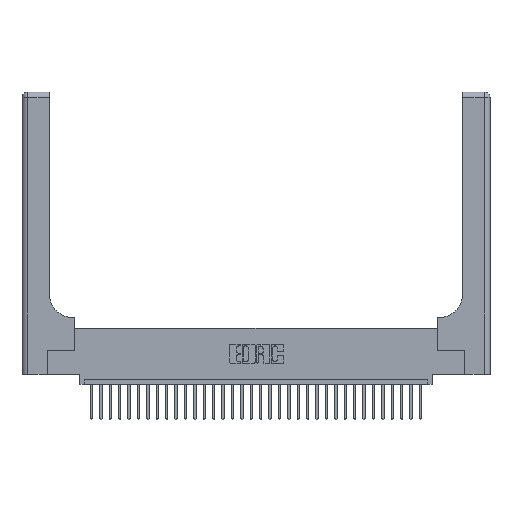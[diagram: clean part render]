
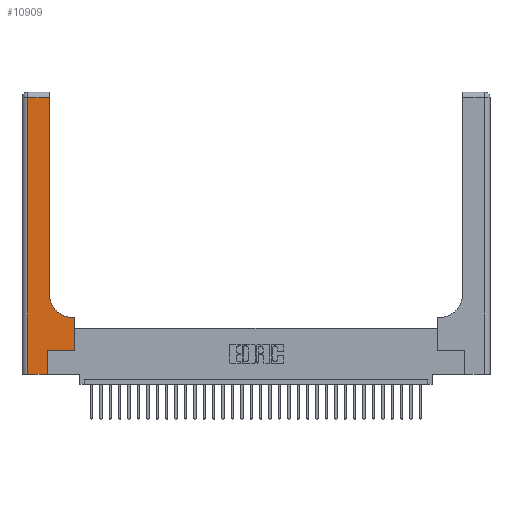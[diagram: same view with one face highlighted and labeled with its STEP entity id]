
A CAD part, top view. The second image highlights one B-rep face of the part: STEP entity #10909.
In plain terms, the highlighted planar face has unit normal (0, 0, 1).
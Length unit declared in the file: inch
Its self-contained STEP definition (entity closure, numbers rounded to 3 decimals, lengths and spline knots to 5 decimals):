
#302 = DIRECTION ( 'NONE',  ( -1., 0., 0. ) ) ;
#313 = CARTESIAN_POINT ( 'NONE',  ( 0., 0., 0.37 ) ) ;
#1082 = DIRECTION ( 'NONE',  ( 0., 1., 0. ) ) ;
#1870 = DIRECTION ( 'NONE',  ( 0., 0., -1. ) ) ;
#2086 = PLANE ( 'NONE',  #30559 ) ;
#2794 = DIRECTION ( 'NONE',  ( 1., 0., 0. ) ) ;
#3475 = VECTOR ( 'NONE', #12350, 39.37008 ) ;
#3550 = VERTEX_POINT ( 'NONE', #29583 ) ;
#3606 = EDGE_CURVE ( 'NONE', #26972, #3550, #19861, .T. ) ;
#3773 = EDGE_CURVE ( 'NONE', #23909, #29468, #15411, .T. ) ;
#4228 = ORIENTED_EDGE ( 'NONE', *, *, #3606, .T. ) ;
#4654 = CARTESIAN_POINT ( 'NONE',  ( 0., 3., 0.37 ) ) ;
#5030 = ORIENTED_EDGE ( 'NONE', *, *, #11536, .T. ) ;
#5395 = DIRECTION ( 'NONE',  ( 0., 1., 0. ) ) ;
#5443 = VECTOR ( 'NONE', #5395, 39.37008 ) ;
#6103 = ORIENTED_EDGE ( 'NONE', *, *, #27163, .T. ) ;
#7341 = DIRECTION ( 'NONE',  ( -1., 0., 0. ) ) ;
#7706 = CARTESIAN_POINT ( 'NONE',  ( 0.269, 0.25, 0.37 ) ) ;
#8297 = CARTESIAN_POINT ( 'NONE',  ( 0.2915, 0.85, 0.37 ) ) ;
#8334 = CARTESIAN_POINT ( 'NONE',  ( 0.5415, 0.85, 0.37 ) ) ;
#8568 = CARTESIAN_POINT ( 'NONE',  ( 0.269, 0., 0.37 ) ) ;
#9108 = CARTESIAN_POINT ( 'NONE',  ( 0.06, 2.94, 0.37 ) ) ;
#9477 = VECTOR ( 'NONE', #7341, 39.37008 ) ;
#9943 = LINE ( 'NONE', #11959, #5443 ) ;
#10534 = LINE ( 'NONE', #15689, #28540 ) ;
#10909 = ADVANCED_FACE ( 'NONE', ( #15616 ), #2086, .F. ) ;
#11064 = VECTOR ( 'NONE', #1082, 39.37008 ) ;
#11536 = EDGE_CURVE ( 'NONE', #12377, #16761, #32868, .T. ) ;
#11605 = EDGE_CURVE ( 'NONE', #32882, #12377, #17578, .T. ) ;
#11951 = LINE ( 'NONE', #15032, #3475 ) ;
#11959 = CARTESIAN_POINT ( 'NONE',  ( 0.269, 0., 0.37 ) ) ;
#12200 = EDGE_CURVE ( 'NONE', #17637, #17462, #11951, .T. ) ;
#12301 = CARTESIAN_POINT ( 'NONE',  ( 0.5585, 0.25, 0.37 ) ) ;
#12350 = DIRECTION ( 'NONE',  ( 1., 0., 0. ) ) ;
#12377 = VERTEX_POINT ( 'NONE', #21167 ) ;
#12618 = EDGE_CURVE ( 'NONE', #16761, #17637, #9943, .T. ) ;
#14243 = EDGE_CURVE ( 'NONE', #3550, #23909, #27149, .T. ) ;
#15032 = CARTESIAN_POINT ( 'NONE',  ( 0.269, 0.25, 0.37 ) ) ;
#15411 = LINE ( 'NONE', #21137, #20235 ) ;
#15616 = FACE_OUTER_BOUND ( 'NONE', #30904, .T. ) ;
#15689 = CARTESIAN_POINT ( 'NONE',  ( 0., 2.94, 0.37 ) ) ;
#15987 = CARTESIAN_POINT ( 'NONE',  ( 0.5585, 0.25, 0.37 ) ) ;
#16761 = VERTEX_POINT ( 'NONE', #8568 ) ;
#17462 = VERTEX_POINT ( 'NONE', #12301 ) ;
#17578 = LINE ( 'NONE', #23060, #28810 ) ;
#17637 = VERTEX_POINT ( 'NONE', #7706 ) ;
#17862 = LINE ( 'NONE', #15987, #11064 ) ;
#19861 = LINE ( 'NONE', #27658, #9477 ) ;
#20159 = ORIENTED_EDGE ( 'NONE', *, *, #29203, .T. ) ;
#20235 = VECTOR ( 'NONE', #30074, 39.37008 ) ;
#20959 = DIRECTION ( 'NONE',  ( 0., 0., -1. ) ) ;
#21137 = CARTESIAN_POINT ( 'NONE',  ( 0.2915, 3., 0.37 ) ) ;
#21167 = CARTESIAN_POINT ( 'NONE',  ( 0.06, 0., 0.37 ) ) ;
#21860 = ORIENTED_EDGE ( 'NONE', *, *, #12618, .T. ) ;
#22401 = DIRECTION ( 'NONE',  ( -1., 0., 0. ) ) ;
#22810 = VECTOR ( 'NONE', #2794, 39.37008 ) ;
#23060 = CARTESIAN_POINT ( 'NONE',  ( 0.06, 3., 0.37 ) ) ;
#23105 = ORIENTED_EDGE ( 'NONE', *, *, #12200, .T. ) ;
#23625 = ORIENTED_EDGE ( 'NONE', *, *, #3773, .T. ) ;
#23909 = VERTEX_POINT ( 'NONE', #8297 ) ;
#26326 = ORIENTED_EDGE ( 'NONE', *, *, #11605, .T. ) ;
#26972 = VERTEX_POINT ( 'NONE', #30841 ) ;
#27044 = CARTESIAN_POINT ( 'NONE',  ( 0.2915, 2.94, 0.37 ) ) ;
#27149 = CIRCLE ( 'NONE', #29766, 0.25 ) ;
#27163 = EDGE_CURVE ( 'NONE', #17462, #26972, #17862, .T. ) ;
#27658 = CARTESIAN_POINT ( 'NONE',  ( 0.2915, 0.6, 0.37 ) ) ;
#28540 = VECTOR ( 'NONE', #302, 39.37008 ) ;
#28810 = VECTOR ( 'NONE', #30820, 39.37008 ) ;
#29203 = EDGE_CURVE ( 'NONE', #29468, #32882, #10534, .T. ) ;
#29468 = VERTEX_POINT ( 'NONE', #27044 ) ;
#29583 = CARTESIAN_POINT ( 'NONE',  ( 0.5415, 0.6, 0.37 ) ) ;
#29766 = AXIS2_PLACEMENT_3D ( 'NONE', #8334, #20959, #31101 ) ;
#30074 = DIRECTION ( 'NONE',  ( 0., 1., 0. ) ) ;
#30559 = AXIS2_PLACEMENT_3D ( 'NONE', #4654, #1870, #22401 ) ;
#30820 = DIRECTION ( 'NONE',  ( 0., -1., 0. ) ) ;
#30841 = CARTESIAN_POINT ( 'NONE',  ( 0.5585, 0.6, 0.37 ) ) ;
#30904 = EDGE_LOOP ( 'NONE', ( #23625, #20159, #26326, #5030, #21860, #23105, #6103, #4228, #32286 ) ) ;
#31101 = DIRECTION ( 'NONE',  ( 1., 0., 0. ) ) ;
#32286 = ORIENTED_EDGE ( 'NONE', *, *, #14243, .T. ) ;
#32868 = LINE ( 'NONE', #313, #22810 ) ;
#32882 = VERTEX_POINT ( 'NONE', #9108 ) ;
